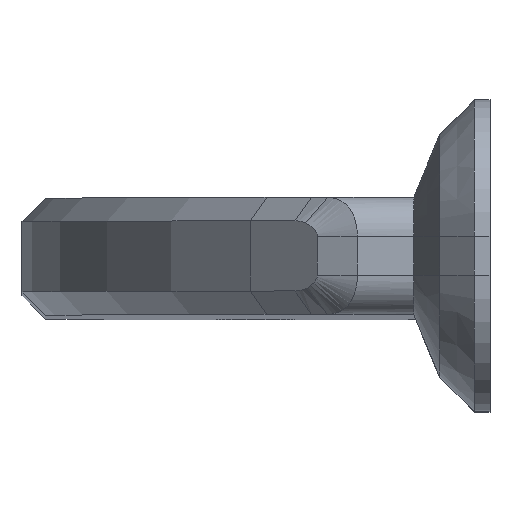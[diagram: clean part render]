
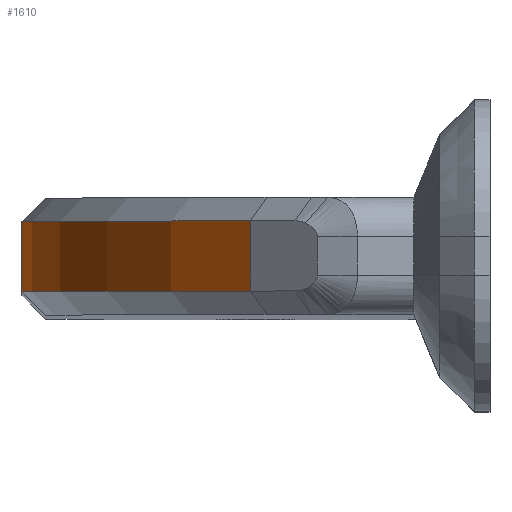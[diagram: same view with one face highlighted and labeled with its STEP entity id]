
A CAD part, top view. The second image highlights one B-rep face of the part: STEP entity #1610.
In plain terms, the highlighted cylindrical face has radius 20 mm (diameter 40 mm), a partial arc.
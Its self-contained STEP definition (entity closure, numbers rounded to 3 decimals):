
#187 = PLANE('',#188);
#188 = AXIS2_PLACEMENT_3D('',#189,#190,#191);
#189 = CARTESIAN_POINT('',(5.,0.,52.308));
#190 = DIRECTION('',(-1.,-0.,0.));
#191 = DIRECTION('',(0.,0.,-1.));
#567 = EDGE_CURVE('',#568,#570,#572,.T.);
#568 = VERTEX_POINT('',#569);
#569 = CARTESIAN_POINT('',(5.,-0.9,80.716));
#570 = VERTEX_POINT('',#571);
#571 = CARTESIAN_POINT('',(5.,0.9,80.716));
#572 = SURFACE_CURVE('',#573,(#577,#584),.PCURVE_S1.);
#573 = LINE('',#574,#575);
#574 = CARTESIAN_POINT('',(5.,-1.5,80.716));
#575 = VECTOR('',#576,1.);
#576 = DIRECTION('',(0.,1.,0.));
#577 = PCURVE('',#187,#578);
#578 = DEFINITIONAL_REPRESENTATION('',(#579),#583);
#579 = LINE('',#580,#581);
#580 = CARTESIAN_POINT('',(-28.408,1.5));
#581 = VECTOR('',#582,1.);
#582 = DIRECTION('',(0.,-1.));
#583 = ( GEOMETRIC_REPRESENTATION_CONTEXT(2) 
PARAMETRIC_REPRESENTATION_CONTEXT() REPRESENTATION_CONTEXT('2D SPACE',''
  ) );
#584 = PCURVE('',#585,#590);
#585 = CYLINDRICAL_SURFACE('',#586,20.);
#586 = AXIS2_PLACEMENT_3D('',#587,#588,#589);
#587 = CARTESIAN_POINT('',(25.,-1.5,80.716));
#588 = DIRECTION('',(0.,1.,0.));
#589 = DIRECTION('',(-1.,0.,0.));
#590 = DEFINITIONAL_REPRESENTATION('',(#591),#595);
#591 = LINE('',#592,#593);
#592 = CARTESIAN_POINT('',(0.,0.));
#593 = VECTOR('',#594,1.);
#594 = DIRECTION('',(0.,1.));
#595 = ( GEOMETRIC_REPRESENTATION_CONTEXT(2) 
PARAMETRIC_REPRESENTATION_CONTEXT() REPRESENTATION_CONTEXT('2D SPACE',''
  ) );
#815 = CONICAL_SURFACE('',#816,20.,0.785);
#816 = AXIS2_PLACEMENT_3D('',#817,#818,#819);
#817 = CARTESIAN_POINT('',(25.,-0.9,80.716));
#818 = DIRECTION('',(0.,1.,0.));
#819 = DIRECTION('',(-0.707,0.,0.707));
#1161 = CONICAL_SURFACE('',#1162,20.,0.785);
#1162 = AXIS2_PLACEMENT_3D('',#1163,#1164,#1165);
#1163 = CARTESIAN_POINT('',(25.,0.9,80.716));
#1164 = DIRECTION('',(0.,-1.,0.));
#1165 = DIRECTION('',(-1.,-0.,0.));
#1610 = ADVANCED_FACE('',(#1611),#585,.T.);
#1611 = FACE_BOUND('',#1612,.T.);
#1612 = EDGE_LOOP('',(#1613,#1643,#1665,#1666));
#1613 = ORIENTED_EDGE('',*,*,#1614,.T.);
#1614 = EDGE_CURVE('',#1615,#1617,#1619,.T.);
#1615 = VERTEX_POINT('',#1616);
#1616 = CARTESIAN_POINT('',(10.858,-0.9,94.858));
#1617 = VERTEX_POINT('',#1618);
#1618 = CARTESIAN_POINT('',(10.858,0.9,94.858));
#1619 = SURFACE_CURVE('',#1620,(#1624,#1631),.PCURVE_S1.);
#1620 = LINE('',#1621,#1622);
#1621 = CARTESIAN_POINT('',(10.858,-1.5,94.858));
#1622 = VECTOR('',#1623,1.);
#1623 = DIRECTION('',(0.,1.,0.));
#1624 = PCURVE('',#585,#1625);
#1625 = DEFINITIONAL_REPRESENTATION('',(#1626),#1630);
#1626 = LINE('',#1627,#1628);
#1627 = CARTESIAN_POINT('',(0.785,0.));
#1628 = VECTOR('',#1629,1.);
#1629 = DIRECTION('',(0.,1.));
#1630 = ( GEOMETRIC_REPRESENTATION_CONTEXT(2) 
PARAMETRIC_REPRESENTATION_CONTEXT() REPRESENTATION_CONTEXT('2D SPACE',''
  ) );
#1631 = PCURVE('',#1632,#1637);
#1632 = PLANE('',#1633);
#1633 = AXIS2_PLACEMENT_3D('',#1634,#1635,#1636);
#1634 = CARTESIAN_POINT('',(9.,-1.5,93.));
#1635 = DIRECTION('',(0.707,0.,-0.707));
#1636 = DIRECTION('',(0.,1.,0.));
#1637 = DEFINITIONAL_REPRESENTATION('',(#1638),#1642);
#1638 = LINE('',#1639,#1640);
#1639 = CARTESIAN_POINT('',(0.,2.627));
#1640 = VECTOR('',#1641,1.);
#1641 = DIRECTION('',(1.,0.));
#1642 = ( GEOMETRIC_REPRESENTATION_CONTEXT(2) 
PARAMETRIC_REPRESENTATION_CONTEXT() REPRESENTATION_CONTEXT('2D SPACE',''
  ) );
#1643 = ORIENTED_EDGE('',*,*,#1644,.F.);
#1644 = EDGE_CURVE('',#570,#1617,#1645,.T.);
#1645 = SURFACE_CURVE('',#1646,(#1651,#1658),.PCURVE_S1.);
#1646 = CIRCLE('',#1647,20.);
#1647 = AXIS2_PLACEMENT_3D('',#1648,#1649,#1650);
#1648 = CARTESIAN_POINT('',(25.,0.9,80.716));
#1649 = DIRECTION('',(0.,1.,-0.));
#1650 = DIRECTION('',(-1.,-0.,0.));
#1651 = PCURVE('',#585,#1652);
#1652 = DEFINITIONAL_REPRESENTATION('',(#1653),#1657);
#1653 = LINE('',#1654,#1655);
#1654 = CARTESIAN_POINT('',(0.,2.4));
#1655 = VECTOR('',#1656,1.);
#1656 = DIRECTION('',(1.,0.));
#1657 = ( GEOMETRIC_REPRESENTATION_CONTEXT(2) 
PARAMETRIC_REPRESENTATION_CONTEXT() REPRESENTATION_CONTEXT('2D SPACE',''
  ) );
#1658 = PCURVE('',#1161,#1659);
#1659 = DEFINITIONAL_REPRESENTATION('',(#1660),#1664);
#1660 = LINE('',#1661,#1662);
#1661 = CARTESIAN_POINT('',(-0.,-0.));
#1662 = VECTOR('',#1663,1.);
#1663 = DIRECTION('',(-1.,-0.));
#1664 = ( GEOMETRIC_REPRESENTATION_CONTEXT(2) 
PARAMETRIC_REPRESENTATION_CONTEXT() REPRESENTATION_CONTEXT('2D SPACE',''
  ) );
#1665 = ORIENTED_EDGE('',*,*,#567,.F.);
#1666 = ORIENTED_EDGE('',*,*,#1667,.F.);
#1667 = EDGE_CURVE('',#1615,#568,#1668,.T.);
#1668 = SURFACE_CURVE('',#1669,(#1674,#1681),.PCURVE_S1.);
#1669 = CIRCLE('',#1670,20.);
#1670 = AXIS2_PLACEMENT_3D('',#1671,#1672,#1673);
#1671 = CARTESIAN_POINT('',(25.,-0.9,80.716));
#1672 = DIRECTION('',(-0.,-1.,0.));
#1673 = DIRECTION('',(-0.707,0.,0.707));
#1674 = PCURVE('',#585,#1675);
#1675 = DEFINITIONAL_REPRESENTATION('',(#1676),#1680);
#1676 = LINE('',#1677,#1678);
#1677 = CARTESIAN_POINT('',(0.785,0.6));
#1678 = VECTOR('',#1679,1.);
#1679 = DIRECTION('',(-1.,-0.));
#1680 = ( GEOMETRIC_REPRESENTATION_CONTEXT(2) 
PARAMETRIC_REPRESENTATION_CONTEXT() REPRESENTATION_CONTEXT('2D SPACE',''
  ) );
#1681 = PCURVE('',#815,#1682);
#1682 = DEFINITIONAL_REPRESENTATION('',(#1683),#1687);
#1683 = LINE('',#1684,#1685);
#1684 = CARTESIAN_POINT('',(-0.,-0.));
#1685 = VECTOR('',#1686,1.);
#1686 = DIRECTION('',(-1.,-0.));
#1687 = ( GEOMETRIC_REPRESENTATION_CONTEXT(2) 
PARAMETRIC_REPRESENTATION_CONTEXT() REPRESENTATION_CONTEXT('2D SPACE',''
  ) );
